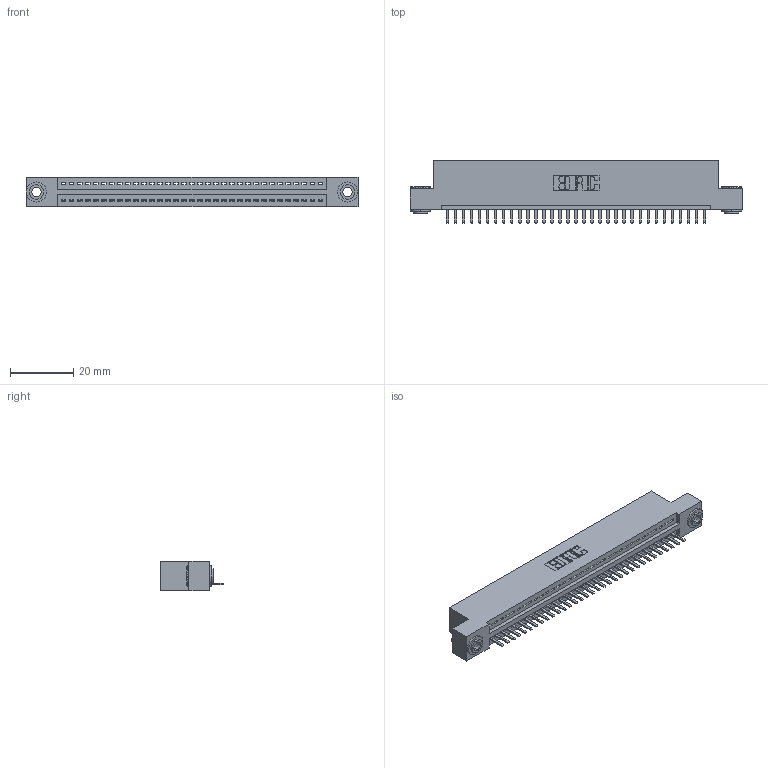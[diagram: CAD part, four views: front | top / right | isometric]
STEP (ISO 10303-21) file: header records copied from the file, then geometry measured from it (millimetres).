
FILE_DESCRIPTION (( 'STEP AP203' ), '1' );
FILE_NAME ('395-033-520-103.STEP', '2019-10-19T15:08:42', ( '' ), ( '' ), 'SwSTEP 2.0', 'SolidWorks 2016', '' );
FILE_SCHEMA (( 'CONFIG_CONTROL_DESIGN' ));
Length unit declared in the file: inch
Products named in the file (4): 345 Part_Flush Mounting Lugs - 0.156 Dia-TH; 345-292-001_345-293-120; 345-250-002_345-250-002-102; 395-033-520-103
Assembly tree (36 placements, depth 2):
  395-033-520-103
    345 Part_Flush Mounting Lugs - 0.156 Dia-TH
    345-292-001_345-293-120  x33
    345-250-002_345-250-002-102  x2
Bounding box: 105.03 x 19.68 x 9.4 mm (x, y, z)
Volume: 9826.5 mm3; surface area: 12840.2 mm2
Topology: 36 solids, 36 shells, 2210 faces, 6489 edges, 4234 vertices
Faces by surface type: plane 1476, cylinder 726, cone 8
Entity records: 26812 total; most frequent: CARTESIAN_POINT 4634, ORIENTED_EDGE 4582, DIRECTION 4079, EDGE_CURVE 2291, VECTOR 1999, LINE 1999, VERTEX_POINT 1522, AXIS2_PLACEMENT_3D 1040
